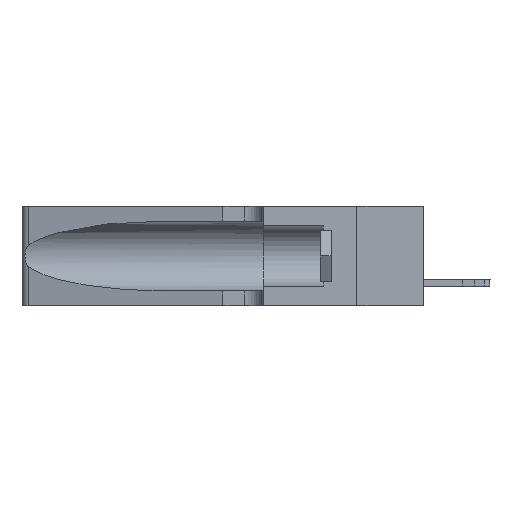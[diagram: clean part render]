
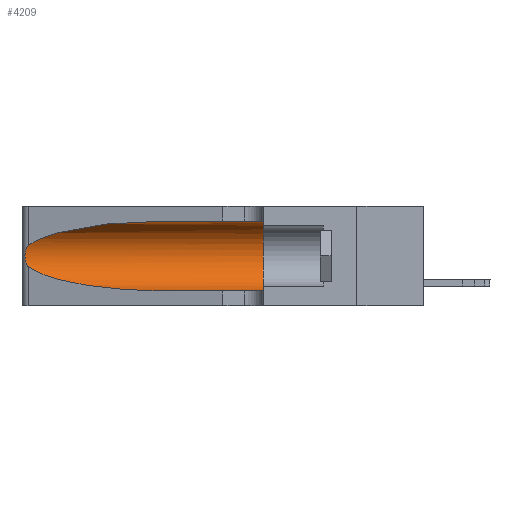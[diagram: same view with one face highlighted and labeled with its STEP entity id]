
A CAD part, left-side view. The second image highlights one B-rep face of the part: STEP entity #4209.
In plain terms, the highlighted cylindrical face has radius 3.308 mm (diameter 6.617 mm), a partial arc.
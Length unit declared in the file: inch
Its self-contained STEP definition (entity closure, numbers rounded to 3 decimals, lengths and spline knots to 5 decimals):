
#450 = CARTESIAN_POINT ( 'NONE',  ( 0.18966, 0.96281, 0.05475 ) ) ;
#469 = DIRECTION ( 'NONE',  ( 0., -1., 0. ) ) ;
#484 = CARTESIAN_POINT ( 'NONE',  ( 0.25856, 1.23593, 0.16098 ) ) ;
#1282 = DIRECTION ( 'NONE',  ( 0., 0., -1. ) ) ;
#1305 = CARTESIAN_POINT ( 'NONE',  ( 0.1305, 1.61858, 0.31525 ) ) ;
#1540 = CARTESIAN_POINT ( 'NONE',  ( 0.1305, 0.35, 0.05475 ) ) ;
#1681 = EDGE_CURVE ( 'NONE', #17236, #13518, #13883, .T. ) ;
#1893 = CARTESIAN_POINT ( 'NONE',  ( 0.25555, 1.22993, 0.14849 ) ) ;
#2057 = CARTESIAN_POINT ( 'NONE',  ( 0.2373, 1.15595, 0.28018 ) ) ;
#2189 = CARTESIAN_POINT ( 'NONE',  ( 0.25487, 1.22718, 0.22369 ) ) ;
#3121 = VECTOR ( 'NONE', #469, 39.37008 ) ;
#3191 = CARTESIAN_POINT ( 'NONE',  ( 0.1305, 1.61858, 0.05475 ) ) ;
#3346 = LINE ( 'NONE', #3191, #3121 ) ;
#3461 = DIRECTION ( 'NONE',  ( 0., 0., 1. ) ) ;
#3524 = LINE ( 'NONE', #1305, #6330 ) ;
#3575 = EDGE_LOOP ( 'NONE', ( #4865, #14564, #3909, #9558, #15985, #10763 ) ) ;
#3577 = CARTESIAN_POINT ( 'NONE',  ( 0.25487, 1.22718, 0.14631 ) ) ;
#3714 = CYLINDRICAL_SURFACE ( 'NONE', #5564, 0.13025 ) ;
#3748 = AXIS2_PLACEMENT_3D ( 'NONE', #10630, #8835, #3461 ) ;
#3909 = ORIENTED_EDGE ( 'NONE', *, *, #1681, .T. ) ;
#3939 = VERTEX_POINT ( 'NONE', #1540 ) ;
#4209 = ADVANCED_FACE ( 'NONE', ( #10994 ), #3714, .F. ) ;
#4473 = CARTESIAN_POINT ( 'NONE',  ( 0.1305, 0.72297, 0.05475 ) ) ;
#4567 = CARTESIAN_POINT ( 'NONE',  ( 0.26018, 1.23835, 0.19895 ) ) ;
#4673 = CARTESIAN_POINT ( 'NONE',  ( 0.18966, 0.96281, 0.31525 ) ) ;
#4865 = ORIENTED_EDGE ( 'NONE', *, *, #11341, .T. ) ;
#4940 = VERTEX_POINT ( 'NONE', #15491 ) ;
#5564 = AXIS2_PLACEMENT_3D ( 'NONE', #13606, #9441, #1282 ) ;
#6040 = CARTESIAN_POINT ( 'NONE',  ( 0.25639, 1.23186, 0.15144 ) ) ;
#6235 = DIRECTION ( 'NONE',  ( 0., -1., 0. ) ) ;
#6330 = VECTOR ( 'NONE', #6235, 39.37008 ) ;
#6448 = EDGE_CURVE ( 'NONE', #13966, #3939, #7074, .T. ) ;
#7074 = CIRCLE ( 'NONE', #3748, 0.13025 ) ;
#7166 = CARTESIAN_POINT ( 'NONE',  ( 0.25854, 1.2359, 0.20912 ) ) ;
#7197 = CARTESIAN_POINT ( 'NONE',  ( 0.25487, 1.22718, 0.14631 ) ) ;
#7224 = EDGE_CURVE ( 'NONE', #13459, #17236, #9739, .T. ) ;
#8025 = CARTESIAN_POINT ( 'NONE',  ( 0.1305, 0.35, 0.31525 ) ) ;
#8632 = CARTESIAN_POINT ( 'NONE',  ( 0.25787, 1.23484, 0.2124 ) ) ;
#8835 = DIRECTION ( 'NONE',  ( 0., 1., 0. ) ) ;
#9441 = DIRECTION ( 'NONE',  ( 0., -1., 0. ) ) ;
#9558 = ORIENTED_EDGE ( 'NONE', *, *, #13099, .T. ) ;
#9739 = B_SPLINE_CURVE_WITH_KNOTS ( 'NONE', 3,
 ( #10129, #12741, #10011, #8632, #7166, #4567, #11454, #16853, #14118, #484, #16910, #6040, #1893, #10071 ),
 .UNSPECIFIED., .F., .F.,
 ( 4, 2, 2, 2, 2, 2, 4 ),
 ( 0., 0.00027, 0.00053, 0.00107, 0.0016, 0.00187, 0.00214 ),
 .UNSPECIFIED. ) ;
#10011 = CARTESIAN_POINT ( 'NONE',  ( 0.25639, 1.23184, 0.21858 ) ) ;
#10071 = CARTESIAN_POINT ( 'NONE',  ( 0.25487, 1.22718, 0.14631 ) ) ;
#10129 = CARTESIAN_POINT ( 'NONE',  ( 0.25487, 1.22718, 0.22369 ) ) ;
#10630 = CARTESIAN_POINT ( 'NONE',  ( 0.1305, 0.35, 0.185 ) ) ;
#10763 = ORIENTED_EDGE ( 'NONE', *, *, #14626, .F. ) ;
#10994 = FACE_OUTER_BOUND ( 'NONE', #3575, .T. ) ;
#11341 = EDGE_CURVE ( 'NONE', #4940, #13459, #14775, .T. ) ;
#11454 = CARTESIAN_POINT ( 'NONE',  ( 0.26075, 1.23896, 0.19203 ) ) ;
#11611 = CARTESIAN_POINT ( 'NONE',  ( 0.25487, 1.22718, 0.22369 ) ) ;
#12741 = CARTESIAN_POINT ( 'NONE',  ( 0.25555, 1.22994, 0.2215 ) ) ;
#13083 = CARTESIAN_POINT ( 'NONE',  ( 0.1305, 0.72297, 0.31525 ) ) ;
#13099 = EDGE_CURVE ( 'NONE', #13518, #3939, #3346, .T. ) ;
#13459 = VERTEX_POINT ( 'NONE', #2189 ) ;
#13518 = VERTEX_POINT ( 'NONE', #17462 ) ;
#13606 = CARTESIAN_POINT ( 'NONE',  ( 0.1305, 1.61858, 0.185 ) ) ;
#13883 =( BOUNDED_CURVE ( )  B_SPLINE_CURVE ( 3, ( #7197, #15225, #450, #4473 ),
 .UNSPECIFIED., .F., .F. ) 
 B_SPLINE_CURVE_WITH_KNOTS ( ( 4, 4 ),
 ( 3.44316, 4.71239 ),
 .UNSPECIFIED. ) 
 CURVE ( )  GEOMETRIC_REPRESENTATION_ITEM ( )  RATIONAL_B_SPLINE_CURVE ( ( 1., 0.87, 0.87, 1. ) ) 
 REPRESENTATION_ITEM ( '' )  );
#13966 = VERTEX_POINT ( 'NONE', #8025 ) ;
#14118 = CARTESIAN_POINT ( 'NONE',  ( 0.26017, 1.23833, 0.17102 ) ) ;
#14564 = ORIENTED_EDGE ( 'NONE', *, *, #7224, .T. ) ;
#14626 = EDGE_CURVE ( 'NONE', #4940, #13966, #3524, .T. ) ;
#14775 =( BOUNDED_CURVE ( )  B_SPLINE_CURVE ( 3, ( #13083, #4673, #2057, #11611 ),
 .UNSPECIFIED., .F., .T. ) 
 B_SPLINE_CURVE_WITH_KNOTS ( ( 4, 4 ),
 ( 1.5708, 2.84003 ),
 .UNSPECIFIED. ) 
 CURVE ( )  GEOMETRIC_REPRESENTATION_ITEM ( )  RATIONAL_B_SPLINE_CURVE ( ( 1., 0.87, 0.87, 1. ) ) 
 REPRESENTATION_ITEM ( '' )  );
#15225 = CARTESIAN_POINT ( 'NONE',  ( 0.2373, 1.15595, 0.08982 ) ) ;
#15491 = CARTESIAN_POINT ( 'NONE',  ( 0.1305, 0.72297, 0.31525 ) ) ;
#15985 = ORIENTED_EDGE ( 'NONE', *, *, #6448, .F. ) ;
#16853 = CARTESIAN_POINT ( 'NONE',  ( 0.26075, 1.23896, 0.178 ) ) ;
#16910 = CARTESIAN_POINT ( 'NONE',  ( 0.25789, 1.23486, 0.15765 ) ) ;
#17236 = VERTEX_POINT ( 'NONE', #3577 ) ;
#17462 = CARTESIAN_POINT ( 'NONE',  ( 0.1305, 0.72297, 0.05475 ) ) ;
